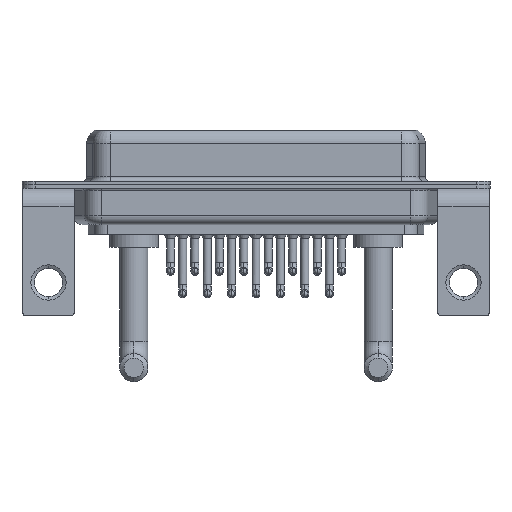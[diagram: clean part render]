
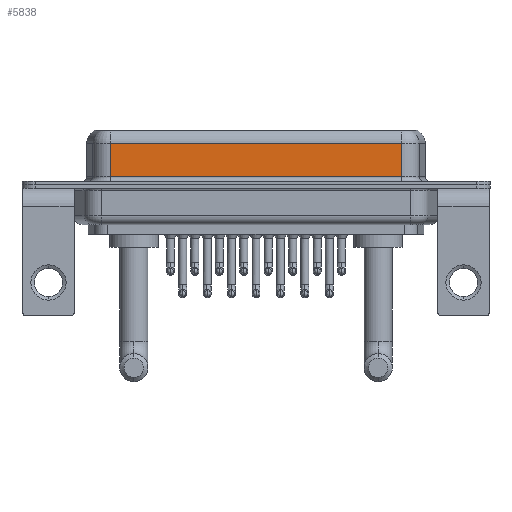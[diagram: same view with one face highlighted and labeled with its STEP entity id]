
A CAD part, front view. The second image highlights one B-rep face of the part: STEP entity #5838.
In plain terms, the highlighted planar face has unit normal (0, -1, 0).
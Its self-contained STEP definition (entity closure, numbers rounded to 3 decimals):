
#655 = VECTOR ( 'NONE', #10033, 1000. ) ;
#1253 = VECTOR ( 'NONE', #10624, 1000. ) ;
#1339 = PLANE ( 'NONE',  #9079 ) ;
#1741 = VERTEX_POINT ( 'NONE', #14462 ) ;
#2041 = LINE ( 'NONE', #16605, #655 ) ;
#2515 = VERTEX_POINT ( 'NONE', #6610 ) ;
#2676 = LINE ( 'NONE', #13829, #6904 ) ;
#2785 = EDGE_LOOP ( 'NONE', ( #3631, #16752, #18354, #16698 ) ) ;
#3631 = ORIENTED_EDGE ( 'NONE', *, *, #14319, .F. ) ;
#4502 = LINE ( 'NONE', #17840, #7718 ) ;
#5058 = EDGE_CURVE ( 'NONE', #2515, #1741, #2041, .T. ) ;
#5838 = ADVANCED_FACE ( 'NONE', ( #16336 ), #1339, .F. ) ;
#6412 = VERTEX_POINT ( 'NONE', #11009 ) ;
#6610 = CARTESIAN_POINT ( 'NONE',  ( 7.013, -3.95, 4.65 ) ) ;
#6904 = VECTOR ( 'NONE', #9143, 1000. ) ;
#7718 = VECTOR ( 'NONE', #16516, 1000. ) ;
#9079 = AXIS2_PLACEMENT_3D ( 'NONE', #19619, #11089, #21259 ) ;
#9143 = DIRECTION ( 'NONE',  ( 0., 0., -1. ) ) ;
#10033 = DIRECTION ( 'NONE',  ( 0., 0., -1. ) ) ;
#10624 = DIRECTION ( 'NONE',  ( 1., 0., 0. ) ) ;
#10934 = CARTESIAN_POINT ( 'NONE',  ( 40.037, -3.95, 4.65 ) ) ;
#10938 = EDGE_CURVE ( 'NONE', #1741, #6412, #15778, .T. ) ;
#11009 = CARTESIAN_POINT ( 'NONE',  ( 40.037, -3.95, 0.9 ) ) ;
#11089 = DIRECTION ( 'NONE',  ( 0., 1., 0. ) ) ;
#11325 = VERTEX_POINT ( 'NONE', #10934 ) ;
#13829 = CARTESIAN_POINT ( 'NONE',  ( 40.037, -3.95, 6.4 ) ) ;
#14319 = EDGE_CURVE ( 'NONE', #11325, #6412, #2676, .T. ) ;
#14462 = CARTESIAN_POINT ( 'NONE',  ( 7.013, -3.95, 0.9 ) ) ;
#15778 = LINE ( 'NONE', #15988, #1253 ) ;
#15988 = CARTESIAN_POINT ( 'NONE',  ( 40.037, -3.95, 0.9 ) ) ;
#16336 = FACE_OUTER_BOUND ( 'NONE', #2785, .T. ) ;
#16516 = DIRECTION ( 'NONE',  ( -1., 0., 0. ) ) ;
#16605 = CARTESIAN_POINT ( 'NONE',  ( 7.013, -3.95, 6.4 ) ) ;
#16698 = ORIENTED_EDGE ( 'NONE', *, *, #10938, .T. ) ;
#16746 = EDGE_CURVE ( 'NONE', #11325, #2515, #4502, .T. ) ;
#16752 = ORIENTED_EDGE ( 'NONE', *, *, #16746, .T. ) ;
#17840 = CARTESIAN_POINT ( 'NONE',  ( 40.037, -3.95, 4.65 ) ) ;
#18354 = ORIENTED_EDGE ( 'NONE', *, *, #5058, .T. ) ;
#19619 = CARTESIAN_POINT ( 'NONE',  ( 40.037, -3.95, 6.4 ) ) ;
#21259 = DIRECTION ( 'NONE',  ( 0., 0., 1. ) ) ;
